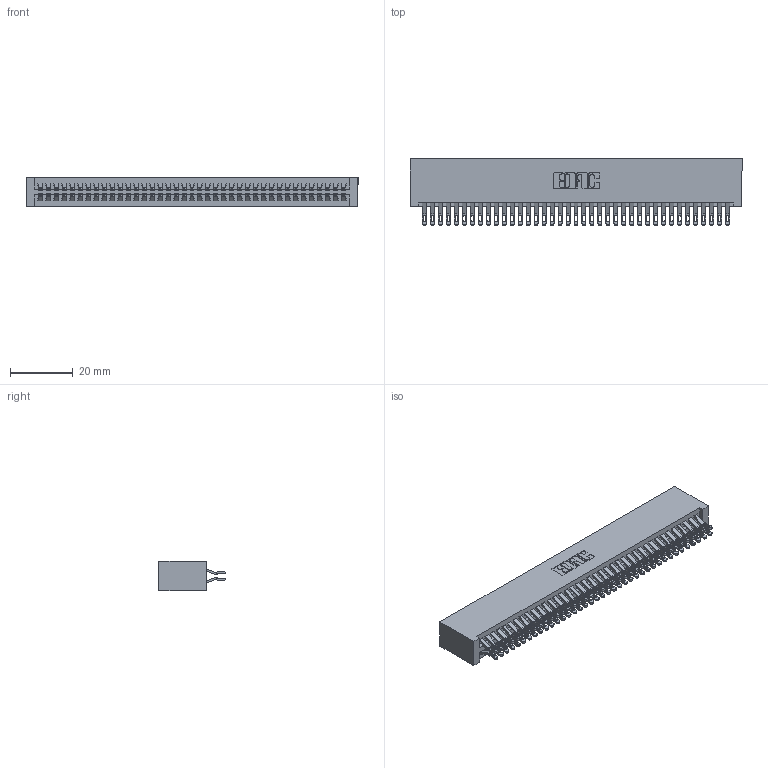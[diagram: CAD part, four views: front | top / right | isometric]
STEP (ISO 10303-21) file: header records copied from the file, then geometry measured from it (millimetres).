
FILE_DESCRIPTION (( 'STEP AP203' ), '1' );
FILE_NAME ('395-078-555-201.STEP', '2019-10-25T02:49:35', ( '' ), ( '' ), 'SwSTEP 2.0', 'SolidWorks 2016', '' );
FILE_SCHEMA (( 'CONFIG_CONTROL_DESIGN' ));
Length unit declared in the file: inch
Products named in the file (3): 345 Part_No Mounting Lugs; 345-292-001_555 Tail; 395-078-555-201
Assembly tree (79 placements, depth 2):
  395-078-555-201
    345 Part_No Mounting Lugs
    345-292-001_555 Tail  x78
Bounding box: 105.66 x 21.13 x 9.4 mm (x, y, z)
Volume: 11078.6 mm3; surface area: 17408.1 mm2
Topology: 79 solids, 79 shells, 4486 faces, 14123 edges, 9414 vertices
Faces by surface type: plane 2494, cylinder 1992
Entity records: 31053 total; most frequent: CARTESIAN_POINT 5242, ORIENTED_EDGE 5146, DIRECTION 4589, EDGE_CURVE 2573, LINE 2273, VECTOR 2273, VERTEX_POINT 1714, AXIS2_PLACEMENT_3D 1158
